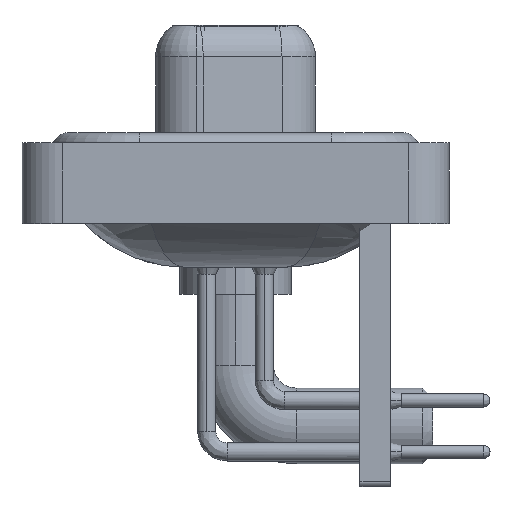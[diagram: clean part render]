
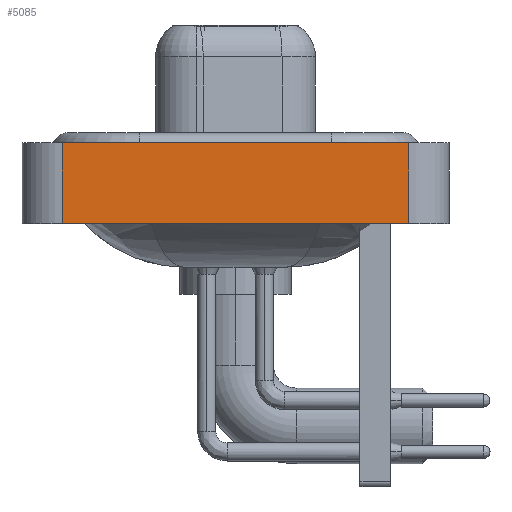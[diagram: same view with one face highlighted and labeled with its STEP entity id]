
A CAD part, left-side view. The second image highlights one B-rep face of the part: STEP entity #5085.
In plain terms, the highlighted planar face has unit normal (-1, 0, 0).
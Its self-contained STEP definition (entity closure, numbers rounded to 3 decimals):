
#270 = CARTESIAN_POINT ( 'NONE',  ( -7.35, -8.55, -3.6 ) ) ;
#774 = EDGE_LOOP ( 'NONE', ( #26322, #25253, #21461, #21435 ) ) ;
#1072 = VERTEX_POINT ( 'NONE', #21736 ) ;
#3434 = DIRECTION ( 'NONE',  ( 0., 0., 1. ) ) ;
#3562 = CARTESIAN_POINT ( 'NONE',  ( -7.35, 8.55, -3.6 ) ) ;
#4115 = VERTEX_POINT ( 'NONE', #6988 ) ;
#4206 = VERTEX_POINT ( 'NONE', #19693 ) ;
#4526 = VECTOR ( 'NONE', #27039, 1000. ) ;
#5085 = ADVANCED_FACE ( 'NONE', ( #26740 ), #5744, .T. ) ;
#5104 = DIRECTION ( 'NONE',  ( 0., -1., 0. ) ) ;
#5647 = VERTEX_POINT ( 'NONE', #270 ) ;
#5665 = LINE ( 'NONE', #3562, #15680 ) ;
#5744 = PLANE ( 'NONE',  #20926 ) ;
#5884 = DIRECTION ( 'NONE',  ( -1., 0., 0. ) ) ;
#6815 = EDGE_CURVE ( 'NONE', #1072, #4206, #13880, .T. ) ;
#6988 = CARTESIAN_POINT ( 'NONE',  ( -7.35, 8.55, -3.6 ) ) ;
#7414 = VECTOR ( 'NONE', #15678, 1000. ) ;
#7677 = DIRECTION ( 'NONE',  ( 0., 0., 1. ) ) ;
#9534 = VECTOR ( 'NONE', #5104, 1000. ) ;
#10865 = EDGE_CURVE ( 'NONE', #4115, #1072, #5665, .T. ) ;
#11071 = EDGE_CURVE ( 'NONE', #4115, #5647, #12558, .T. ) ;
#12558 = LINE ( 'NONE', #21642, #9534 ) ;
#13880 = LINE ( 'NONE', #21730, #7414 ) ;
#14486 = CARTESIAN_POINT ( 'NONE',  ( -7.35, -8.55, -3.6 ) ) ;
#15417 = EDGE_CURVE ( 'NONE', #5647, #4206, #20685, .T. ) ;
#15678 = DIRECTION ( 'NONE',  ( 0., -1., 0. ) ) ;
#15680 = VECTOR ( 'NONE', #3434, 1000. ) ;
#19693 = CARTESIAN_POINT ( 'NONE',  ( -7.35, -8.55, 0.4 ) ) ;
#20685 = LINE ( 'NONE', #14486, #4526 ) ;
#20926 = AXIS2_PLACEMENT_3D ( 'NONE', #27125, #5884, #7677 ) ;
#21435 = ORIENTED_EDGE ( 'NONE', *, *, #11071, .T. ) ;
#21461 = ORIENTED_EDGE ( 'NONE', *, *, #10865, .F. ) ;
#21642 = CARTESIAN_POINT ( 'NONE',  ( -7.35, -8.55, -3.6 ) ) ;
#21730 = CARTESIAN_POINT ( 'NONE',  ( -7.35, -8.55, 0.4 ) ) ;
#21736 = CARTESIAN_POINT ( 'NONE',  ( -7.35, 8.55, 0.4 ) ) ;
#25253 = ORIENTED_EDGE ( 'NONE', *, *, #6815, .F. ) ;
#26322 = ORIENTED_EDGE ( 'NONE', *, *, #15417, .T. ) ;
#26740 = FACE_OUTER_BOUND ( 'NONE', #774, .T. ) ;
#27039 = DIRECTION ( 'NONE',  ( 0., 0., 1. ) ) ;
#27125 = CARTESIAN_POINT ( 'NONE',  ( -7.35, -8.55, -3.6 ) ) ;
